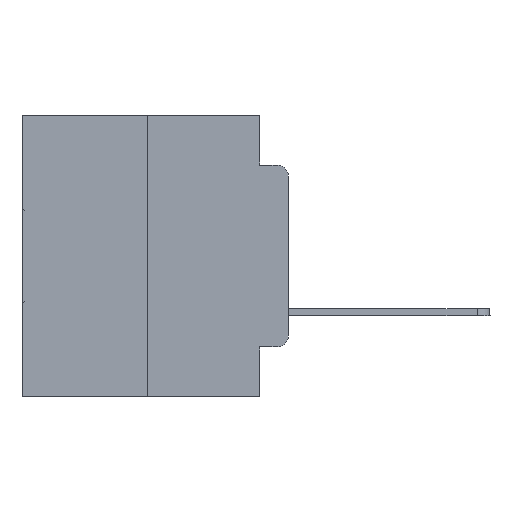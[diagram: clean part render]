
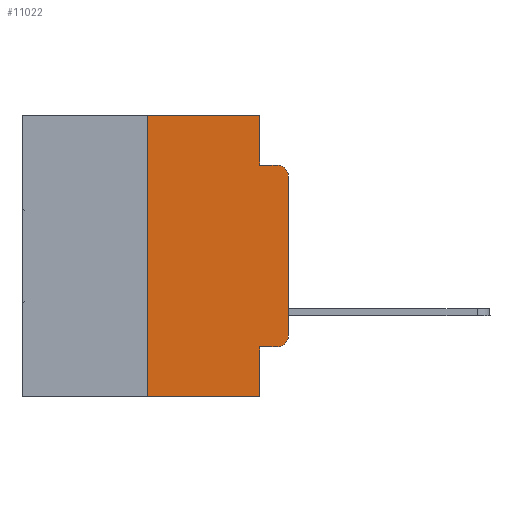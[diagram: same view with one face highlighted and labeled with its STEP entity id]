
A CAD part, left-side view. The second image highlights one B-rep face of the part: STEP entity #11022.
In plain terms, the highlighted planar face has unit normal (-1, 0, 0).
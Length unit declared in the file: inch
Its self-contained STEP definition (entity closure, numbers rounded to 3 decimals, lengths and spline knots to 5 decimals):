
#692 = EDGE_CURVE ( 'NONE', #23234, #13477, #4981, .T. ) ;
#1135 = EDGE_CURVE ( 'NONE', #17736, #23234, #3897, .T. ) ;
#1153 = VERTEX_POINT ( 'NONE', #14357 ) ;
#1861 = DIRECTION ( 'NONE',  ( 0., 0., -1. ) ) ;
#1963 = EDGE_CURVE ( 'NONE', #24765, #19734, #7433, .T. ) ;
#2118 = CARTESIAN_POINT ( 'NONE',  ( 0., 0.051, 0. ) ) ;
#3320 = VECTOR ( 'NONE', #12739, 39.37008 ) ;
#3497 = VECTOR ( 'NONE', #18924, 39.37008 ) ;
#3560 = LINE ( 'NONE', #2118, #14393 ) ;
#3830 = DIRECTION ( 'NONE',  ( 0., 0., -1. ) ) ;
#3897 = LINE ( 'NONE', #16299, #3497 ) ;
#3925 = ORIENTED_EDGE ( 'NONE', *, *, #1135, .T. ) ;
#4112 = CARTESIAN_POINT ( 'NONE',  ( 0., 0.051, -0.0885 ) ) ;
#4567 = LINE ( 'NONE', #11983, #6726 ) ;
#4981 = CIRCLE ( 'NONE', #16704, 0.02 ) ;
#4994 = DIRECTION ( 'NONE',  ( 1., 0., 0. ) ) ;
#5144 = EDGE_CURVE ( 'NONE', #12670, #19734, #8446, .T. ) ;
#5925 = CARTESIAN_POINT ( 'NONE',  ( 0., 0.02, -0.3915 ) ) ;
#6454 = FACE_OUTER_BOUND ( 'NONE', #25871, .T. ) ;
#6521 = VECTOR ( 'NONE', #1861, 39.37008 ) ;
#6726 = VECTOR ( 'NONE', #26021, 39.37008 ) ;
#6778 = ORIENTED_EDGE ( 'NONE', *, *, #26809, .F. ) ;
#7433 = CIRCLE ( 'NONE', #11714, 0.02 ) ;
#7766 = CARTESIAN_POINT ( 'NONE',  ( 0., 0.051, -0.0885 ) ) ;
#8080 = LINE ( 'NONE', #23314, #21846 ) ;
#8390 = DIRECTION ( 'NONE',  ( 0., 0., 1. ) ) ;
#8446 = LINE ( 'NONE', #7766, #3320 ) ;
#9005 = DIRECTION ( 'NONE',  ( -1., 0., 0. ) ) ;
#9089 = VERTEX_POINT ( 'NONE', #29915 ) ;
#9102 = DIRECTION ( 'NONE',  ( 0., 0., -1. ) ) ;
#10303 = EDGE_CURVE ( 'NONE', #13477, #24765, #11574, .T. ) ;
#10362 = CARTESIAN_POINT ( 'NONE',  ( 0., 0.473, -0.5 ) ) ;
#10600 = CARTESIAN_POINT ( 'NONE',  ( 0., 0.02, -0.4115 ) ) ;
#10947 = ORIENTED_EDGE ( 'NONE', *, *, #17132, .T. ) ;
#11022 = ADVANCED_FACE ( 'NONE', ( #6454 ), #11110, .F. ) ;
#11110 = PLANE ( 'NONE',  #12872 ) ;
#11574 = LINE ( 'NONE', #24721, #22484 ) ;
#11714 = AXIS2_PLACEMENT_3D ( 'NONE', #15893, #9005, #9102 ) ;
#11983 = CARTESIAN_POINT ( 'NONE',  ( 0., 0.25, 0. ) ) ;
#12307 = EDGE_CURVE ( 'NONE', #18762, #1153, #4567, .T. ) ;
#12449 = VECTOR ( 'NONE', #26728, 39.37008 ) ;
#12670 = VERTEX_POINT ( 'NONE', #4112 ) ;
#12739 = DIRECTION ( 'NONE',  ( 0., -1., 0. ) ) ;
#12872 = AXIS2_PLACEMENT_3D ( 'NONE', #23461, #4994, #14235 ) ;
#13477 = VERTEX_POINT ( 'NONE', #22322 ) ;
#13619 = ORIENTED_EDGE ( 'NONE', *, *, #27412, .F. ) ;
#14082 = CARTESIAN_POINT ( 'NONE',  ( 0., 0., -0.1085 ) ) ;
#14235 = DIRECTION ( 'NONE',  ( 0., 0., -1. ) ) ;
#14357 = CARTESIAN_POINT ( 'NONE',  ( 0., 0.25, 0. ) ) ;
#14393 = VECTOR ( 'NONE', #22998, 39.37008 ) ;
#15227 = LINE ( 'NONE', #15725, #6521 ) ;
#15725 = CARTESIAN_POINT ( 'NONE',  ( 0., 0.051, 0. ) ) ;
#15893 = CARTESIAN_POINT ( 'NONE',  ( 0., 0.02, -0.1085 ) ) ;
#16299 = CARTESIAN_POINT ( 'NONE',  ( 0., 0.051, -0.4115 ) ) ;
#16704 = AXIS2_PLACEMENT_3D ( 'NONE', #5925, #22184, #3830 ) ;
#17132 = EDGE_CURVE ( 'NONE', #18762, #18652, #26283, .T. ) ;
#17736 = VERTEX_POINT ( 'NONE', #24440 ) ;
#18652 = VERTEX_POINT ( 'NONE', #29374 ) ;
#18737 = CARTESIAN_POINT ( 'NONE',  ( 0., 0.02, -0.0885 ) ) ;
#18762 = VERTEX_POINT ( 'NONE', #27759 ) ;
#18924 = DIRECTION ( 'NONE',  ( 0., -1., 0. ) ) ;
#19734 = VERTEX_POINT ( 'NONE', #18737 ) ;
#21846 = VECTOR ( 'NONE', #22933, 39.37008 ) ;
#22184 = DIRECTION ( 'NONE',  ( -1., 0., 0. ) ) ;
#22322 = CARTESIAN_POINT ( 'NONE',  ( 0., 0., -0.3915 ) ) ;
#22484 = VECTOR ( 'NONE', #8390, 39.37008 ) ;
#22826 = EDGE_CURVE ( 'NONE', #17736, #18652, #15227, .T. ) ;
#22933 = DIRECTION ( 'NONE',  ( 0., -1., 0. ) ) ;
#22998 = DIRECTION ( 'NONE',  ( 0., 0., -1. ) ) ;
#23234 = VERTEX_POINT ( 'NONE', #10600 ) ;
#23314 = CARTESIAN_POINT ( 'NONE',  ( 0., 0.473, 0. ) ) ;
#23461 = CARTESIAN_POINT ( 'NONE',  ( 0., 0.473, 0. ) ) ;
#24440 = CARTESIAN_POINT ( 'NONE',  ( 0., 0.051, -0.4115 ) ) ;
#24721 = CARTESIAN_POINT ( 'NONE',  ( 0., 0., 0. ) ) ;
#24765 = VERTEX_POINT ( 'NONE', #14082 ) ;
#25871 = EDGE_LOOP ( 'NONE', ( #29773, #27993, #28490, #13619, #6778, #27761, #10947, #29760, #3925, #28316 ) ) ;
#26021 = DIRECTION ( 'NONE',  ( 0., 0., 1. ) ) ;
#26283 = LINE ( 'NONE', #10362, #12449 ) ;
#26728 = DIRECTION ( 'NONE',  ( 0., -1., 0. ) ) ;
#26809 = EDGE_CURVE ( 'NONE', #1153, #9089, #8080, .T. ) ;
#27412 = EDGE_CURVE ( 'NONE', #9089, #12670, #3560, .T. ) ;
#27759 = CARTESIAN_POINT ( 'NONE',  ( 0., 0.25, -0.5 ) ) ;
#27761 = ORIENTED_EDGE ( 'NONE', *, *, #12307, .F. ) ;
#27993 = ORIENTED_EDGE ( 'NONE', *, *, #1963, .T. ) ;
#28316 = ORIENTED_EDGE ( 'NONE', *, *, #692, .T. ) ;
#28490 = ORIENTED_EDGE ( 'NONE', *, *, #5144, .F. ) ;
#29374 = CARTESIAN_POINT ( 'NONE',  ( 0., 0.051, -0.5 ) ) ;
#29760 = ORIENTED_EDGE ( 'NONE', *, *, #22826, .F. ) ;
#29773 = ORIENTED_EDGE ( 'NONE', *, *, #10303, .T. ) ;
#29915 = CARTESIAN_POINT ( 'NONE',  ( 0., 0.051, 0. ) ) ;
